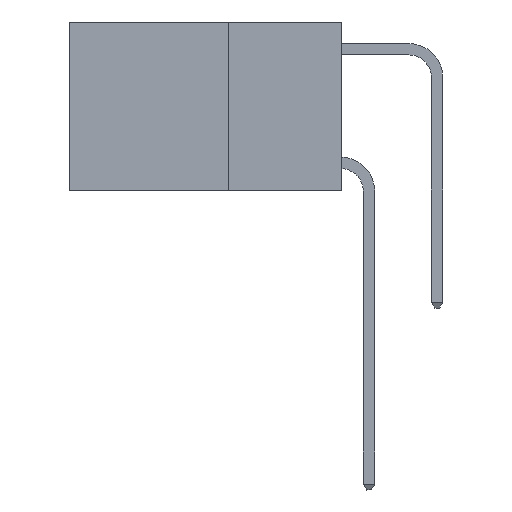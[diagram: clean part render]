
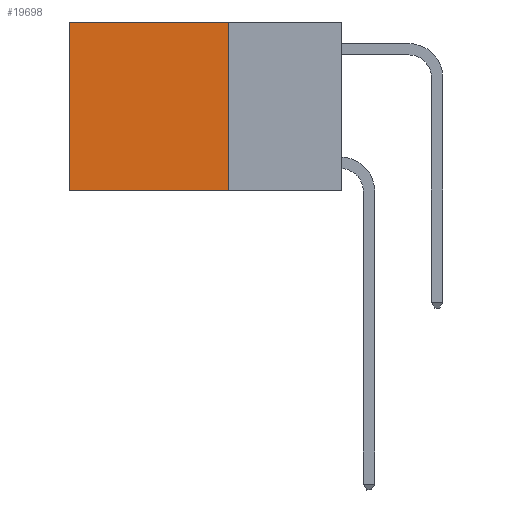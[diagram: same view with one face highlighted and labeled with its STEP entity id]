
A CAD part, left-side view. The second image highlights one B-rep face of the part: STEP entity #19698.
In plain terms, the highlighted planar face has unit normal (-1, 0, 0).
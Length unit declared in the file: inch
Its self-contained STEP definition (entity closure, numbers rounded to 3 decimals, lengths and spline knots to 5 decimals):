
#418 = CARTESIAN_POINT ( 'NONE',  ( 0.2625, 0.25, -0.37 ) ) ;
#602 = VECTOR ( 'NONE', #11499, 39.37008 ) ;
#689 = DIRECTION ( 'NONE',  ( 0., 0., -1. ) ) ;
#949 = EDGE_LOOP ( 'NONE', ( #14130, #15958, #1291, #16469 ) ) ;
#1018 = CARTESIAN_POINT ( 'NONE',  ( 0.2625, 0.25, -0.37 ) ) ;
#1291 = ORIENTED_EDGE ( 'NONE', *, *, #6752, .F. ) ;
#1730 = CARTESIAN_POINT ( 'NONE',  ( 0.2625, 0.25, 0. ) ) ;
#2131 = CARTESIAN_POINT ( 'NONE',  ( 0.2625, 0.25, 0. ) ) ;
#2170 = EDGE_CURVE ( 'NONE', #11259, #4516, #16856, .T. ) ;
#2608 = AXIS2_PLACEMENT_3D ( 'NONE', #5002, #16260, #6648 ) ;
#4167 = LINE ( 'NONE', #18684, #12772 ) ;
#4207 = DIRECTION ( 'NONE',  ( 0., 0., -1. ) ) ;
#4516 = VERTEX_POINT ( 'NONE', #19320 ) ;
#4716 = EDGE_CURVE ( 'NONE', #16733, #4516, #6687, .T. ) ;
#5002 = CARTESIAN_POINT ( 'NONE',  ( 0.2625, 0.25, 0. ) ) ;
#5045 = LINE ( 'NONE', #1730, #602 ) ;
#5700 = CARTESIAN_POINT ( 'NONE',  ( 0.2625, 0.6, 0. ) ) ;
#6648 = DIRECTION ( 'NONE',  ( 0., 0., -1. ) ) ;
#6687 = LINE ( 'NONE', #5700, #14733 ) ;
#6752 = EDGE_CURVE ( 'NONE', #15538, #11259, #4167, .T. ) ;
#7117 = FACE_OUTER_BOUND ( 'NONE', #949, .T. ) ;
#8053 = CARTESIAN_POINT ( 'NONE',  ( 0.2625, 0.6, 0. ) ) ;
#8316 = VECTOR ( 'NONE', #11876, 39.37008 ) ;
#10145 = EDGE_CURVE ( 'NONE', #15538, #16733, #5045, .T. ) ;
#11259 = VERTEX_POINT ( 'NONE', #1018 ) ;
#11499 = DIRECTION ( 'NONE',  ( 0., 1., 0. ) ) ;
#11876 = DIRECTION ( 'NONE',  ( 0., 1., 0. ) ) ;
#12772 = VECTOR ( 'NONE', #4207, 39.37008 ) ;
#14130 = ORIENTED_EDGE ( 'NONE', *, *, #4716, .T. ) ;
#14733 = VECTOR ( 'NONE', #689, 39.37008 ) ;
#15538 = VERTEX_POINT ( 'NONE', #2131 ) ;
#15958 = ORIENTED_EDGE ( 'NONE', *, *, #2170, .F. ) ;
#16260 = DIRECTION ( 'NONE',  ( 1., 0., 0. ) ) ;
#16469 = ORIENTED_EDGE ( 'NONE', *, *, #10145, .T. ) ;
#16631 = PLANE ( 'NONE',  #2608 ) ;
#16733 = VERTEX_POINT ( 'NONE', #8053 ) ;
#16856 = LINE ( 'NONE', #418, #8316 ) ;
#18684 = CARTESIAN_POINT ( 'NONE',  ( 0.2625, 0.25, 0. ) ) ;
#19320 = CARTESIAN_POINT ( 'NONE',  ( 0.2625, 0.6, -0.37 ) ) ;
#19698 = ADVANCED_FACE ( 'NONE', ( #7117 ), #16631, .F. ) ;
